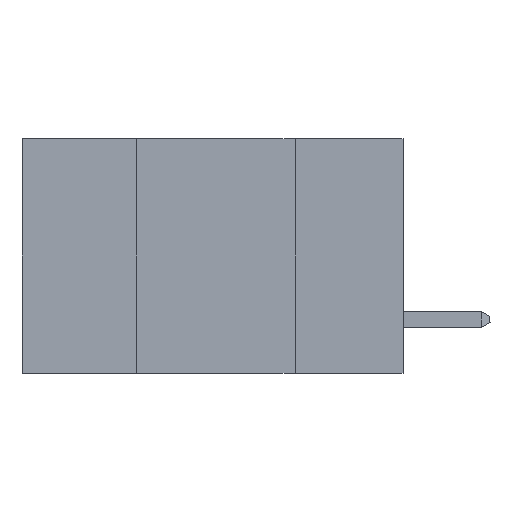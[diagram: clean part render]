
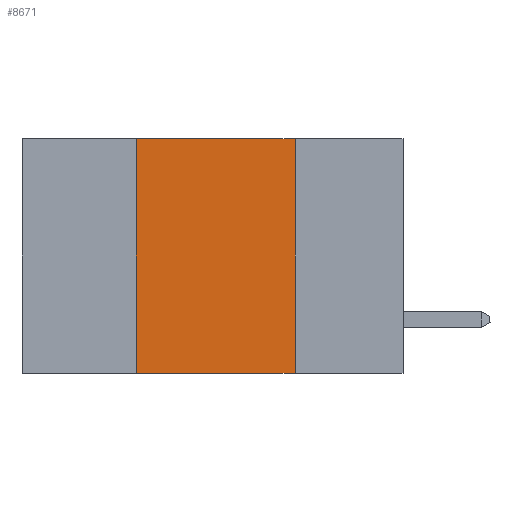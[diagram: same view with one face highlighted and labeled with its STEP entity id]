
A CAD part, left-side view. The second image highlights one B-rep face of the part: STEP entity #8671.
In plain terms, the highlighted planar face has unit normal (-1, 0, 0).
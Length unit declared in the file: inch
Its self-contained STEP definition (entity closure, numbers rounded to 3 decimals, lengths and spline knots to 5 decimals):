
#143 = ORIENTED_EDGE ( 'NONE', *, *, #9811, .F. ) ;
#551 = VECTOR ( 'NONE', #13935, 39.37008 ) ;
#776 = VECTOR ( 'NONE', #18027, 39.37008 ) ;
#3161 = DIRECTION ( 'NONE',  ( 0., 0., -1. ) ) ;
#4033 = CARTESIAN_POINT ( 'NONE',  ( 0., 0.6, 0. ) ) ;
#4335 = FACE_OUTER_BOUND ( 'NONE', #8340, .T. ) ;
#4487 = ORIENTED_EDGE ( 'NONE', *, *, #15449, .F. ) ;
#4675 = DIRECTION ( 'NONE',  ( 0., -1., 0. ) ) ;
#7057 = VERTEX_POINT ( 'NONE', #10037 ) ;
#7396 = VECTOR ( 'NONE', #9014, 39.37008 ) ;
#7438 = PLANE ( 'NONE',  #9998 ) ;
#7807 = LINE ( 'NONE', #4033, #776 ) ;
#8340 = EDGE_LOOP ( 'NONE', ( #143, #4487, #10039, #12986 ) ) ;
#8671 = ADVANCED_FACE ( 'NONE', ( #4335 ), #7438, .F. ) ;
#8706 = LINE ( 'NONE', #9749, #7396 ) ;
#9014 = DIRECTION ( 'NONE',  ( 0., 0., -1. ) ) ;
#9749 = CARTESIAN_POINT ( 'NONE',  ( 0., 0.17, 0. ) ) ;
#9811 = EDGE_CURVE ( 'NONE', #12071, #7057, #8706, .T. ) ;
#9998 = AXIS2_PLACEMENT_3D ( 'NONE', #12884, #14299, #3161 ) ;
#10037 = CARTESIAN_POINT ( 'NONE',  ( 0., 0.17, -0.37 ) ) ;
#10039 = ORIENTED_EDGE ( 'NONE', *, *, #10854, .F. ) ;
#10585 = CARTESIAN_POINT ( 'NONE',  ( 0., 0.42, 0. ) ) ;
#10854 = EDGE_CURVE ( 'NONE', #17171, #13984, #13872, .T. ) ;
#11746 = VECTOR ( 'NONE', #4675, 39.37008 ) ;
#12071 = VERTEX_POINT ( 'NONE', #15291 ) ;
#12884 = CARTESIAN_POINT ( 'NONE',  ( 0., 0.6, 0. ) ) ;
#12902 = CARTESIAN_POINT ( 'NONE',  ( 0., 0.6, -0.37 ) ) ;
#12986 = ORIENTED_EDGE ( 'NONE', *, *, #14478, .T. ) ;
#13821 = CARTESIAN_POINT ( 'NONE',  ( 0., 0.42, 0. ) ) ;
#13872 = LINE ( 'NONE', #13821, #551 ) ;
#13935 = DIRECTION ( 'NONE',  ( 0., 0., 1. ) ) ;
#13984 = VERTEX_POINT ( 'NONE', #10585 ) ;
#14299 = DIRECTION ( 'NONE',  ( 1., 0., 0. ) ) ;
#14478 = EDGE_CURVE ( 'NONE', #17171, #7057, #15416, .T. ) ;
#15291 = CARTESIAN_POINT ( 'NONE',  ( 0., 0.17, 0. ) ) ;
#15416 = LINE ( 'NONE', #12902, #11746 ) ;
#15449 = EDGE_CURVE ( 'NONE', #13984, #12071, #7807, .T. ) ;
#17171 = VERTEX_POINT ( 'NONE', #17177 ) ;
#17177 = CARTESIAN_POINT ( 'NONE',  ( 0., 0.42, -0.37 ) ) ;
#18027 = DIRECTION ( 'NONE',  ( 0., -1., 0. ) ) ;
